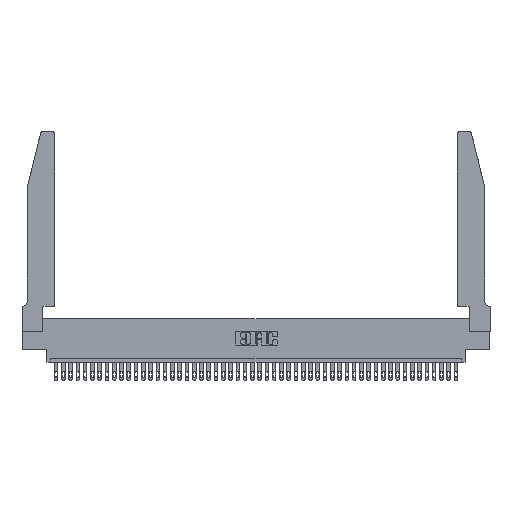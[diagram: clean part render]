
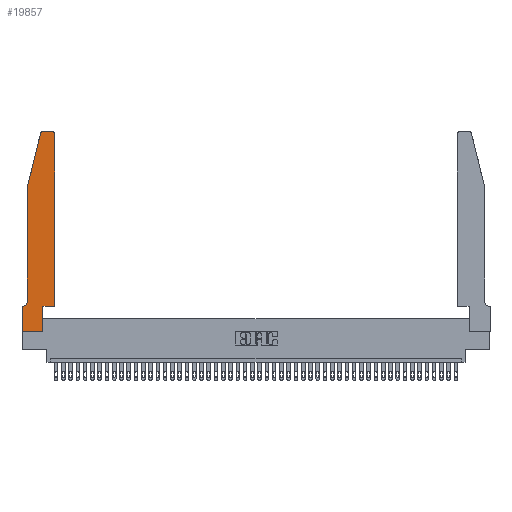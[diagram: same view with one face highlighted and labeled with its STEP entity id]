
A CAD part, top view. The second image highlights one B-rep face of the part: STEP entity #19857.
In plain terms, the highlighted planar face has unit normal (0, 0, 1).
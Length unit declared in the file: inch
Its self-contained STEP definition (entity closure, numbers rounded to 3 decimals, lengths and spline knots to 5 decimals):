
#42 = DIRECTION ( 'NONE',  ( -1., 0., 0. ) ) ;
#402 = CARTESIAN_POINT ( 'NONE',  ( 0.0755, 0.35, 0.37 ) ) ;
#424 = EDGE_CURVE ( 'NONE', #44941, #26855, #13581, .T. ) ;
#565 = EDGE_CURVE ( 'NONE', #4076, #39928, #29343, .T. ) ;
#1055 = CARTESIAN_POINT ( 'NONE',  ( 0., 0., 0.37 ) ) ;
#1721 = VERTEX_POINT ( 'NONE', #27410 ) ;
#1811 = CARTESIAN_POINT ( 'NONE',  ( 0.0055, 0.42, 0.37 ) ) ;
#3792 = ORIENTED_EDGE ( 'NONE', *, *, #565, .T. ) ;
#4076 = VERTEX_POINT ( 'NONE', #27846 ) ;
#5322 = DIRECTION ( 'NONE',  ( -1., 0., 0. ) ) ;
#5922 = VERTEX_POINT ( 'NONE', #16880 ) ;
#6200 = CARTESIAN_POINT ( 'NONE',  ( 0.0755, 2., 0.37 ) ) ;
#6797 = CARTESIAN_POINT ( 'NONE',  ( 0., 0., 0.37 ) ) ;
#7977 = DIRECTION ( 'NONE',  ( 0., 1., 0. ) ) ;
#7980 = LINE ( 'NONE', #35970, #43939 ) ;
#8084 = EDGE_LOOP ( 'NONE', ( #31897, #26178, #3792, #16799, #24186, #38973, #32315, #42271, #27465, #10610, #21210, #30016 ) ) ;
#8278 = DIRECTION ( 'NONE',  ( 0., 0., 1. ) ) ;
#8656 = CARTESIAN_POINT ( 'NONE',  ( 0.2865, 0., 0.37 ) ) ;
#9208 = FACE_OUTER_BOUND ( 'NONE', #8084, .T. ) ;
#9556 = VECTOR ( 'NONE', #25522, 39.37008 ) ;
#10610 = ORIENTED_EDGE ( 'NONE', *, *, #17469, .T. ) ;
#11180 = CARTESIAN_POINT ( 'NONE',  ( 0., 0.35, 0.37 ) ) ;
#11490 = CARTESIAN_POINT ( 'NONE',  ( 0., 0.35, 0.37 ) ) ;
#12446 = DIRECTION ( 'NONE',  ( -1., 0., 0. ) ) ;
#12644 = CIRCLE ( 'NONE', #36156, 0.03 ) ;
#13353 = DIRECTION ( 'NONE',  ( 0., -1., 0. ) ) ;
#13367 = VERTEX_POINT ( 'NONE', #11490 ) ;
#13550 = DIRECTION ( 'NONE',  ( 1., 0., 0. ) ) ;
#13581 = LINE ( 'NONE', #30031, #29385 ) ;
#14349 = DIRECTION ( 'NONE',  ( -0.239, -0.971, 0. ) ) ;
#15126 = DIRECTION ( 'NONE',  ( 0., 1., 0. ) ) ;
#15372 = CIRCLE ( 'NONE', #18150, 0.07 ) ;
#15380 = CARTESIAN_POINT ( 'NONE',  ( 0.0755, 2., 0.37 ) ) ;
#15788 = EDGE_CURVE ( 'NONE', #32384, #19058, #18793, .T. ) ;
#16799 = ORIENTED_EDGE ( 'NONE', *, *, #23053, .T. ) ;
#16880 = CARTESIAN_POINT ( 'NONE',  ( 0.2865, 0.35, 0.37 ) ) ;
#17407 = LINE ( 'NONE', #43301, #25046 ) ;
#17469 = EDGE_CURVE ( 'NONE', #5922, #43700, #27540, .T. ) ;
#18100 = EDGE_CURVE ( 'NONE', #21520, #44941, #12644, .T. ) ;
#18150 = AXIS2_PLACEMENT_3D ( 'NONE', #1811, #26254, #5322 ) ;
#18564 = CARTESIAN_POINT ( 'NONE',  ( 0.4505, 0.35, 0.37 ) ) ;
#18793 = LINE ( 'NONE', #1055, #9556 ) ;
#19058 = VERTEX_POINT ( 'NONE', #8656 ) ;
#19482 = LINE ( 'NONE', #6797, #43342 ) ;
#19632 = EDGE_CURVE ( 'NONE', #19058, #5922, #17407, .T. ) ;
#19857 = ADVANCED_FACE ( 'NONE', ( #9208 ), #25406, .T. ) ;
#20082 = AXIS2_PLACEMENT_3D ( 'NONE', #40966, #23455, #13550 ) ;
#21210 = ORIENTED_EDGE ( 'NONE', *, *, #23343, .T. ) ;
#21415 = CARTESIAN_POINT ( 'NONE',  ( 0.0055, 0.35, 0.37 ) ) ;
#21520 = VERTEX_POINT ( 'NONE', #23321 ) ;
#22359 = CARTESIAN_POINT ( 'NONE',  ( 0., 0., 0.37 ) ) ;
#22390 = DIRECTION ( 'NONE',  ( 0., -1., 0. ) ) ;
#23053 = EDGE_CURVE ( 'NONE', #39928, #1721, #25487, .T. ) ;
#23083 = VECTOR ( 'NONE', #29264, 39.37008 ) ;
#23321 = CARTESIAN_POINT ( 'NONE',  ( 0.4505, 2.72, 0.37 ) ) ;
#23343 = EDGE_CURVE ( 'NONE', #43700, #21520, #7980, .T. ) ;
#23455 = DIRECTION ( 'NONE',  ( 0., 0., 1. ) ) ;
#24186 = ORIENTED_EDGE ( 'NONE', *, *, #42506, .T. ) ;
#25046 = VECTOR ( 'NONE', #7977, 39.37008 ) ;
#25406 = PLANE ( 'NONE',  #39424 ) ;
#25487 = LINE ( 'NONE', #15380, #37453 ) ;
#25522 = DIRECTION ( 'NONE',  ( 1., 0., 0. ) ) ;
#26178 = ORIENTED_EDGE ( 'NONE', *, *, #28301, .T. ) ;
#26254 = DIRECTION ( 'NONE',  ( 0., 0., -1. ) ) ;
#26855 = VERTEX_POINT ( 'NONE', #32047 ) ;
#27380 = DIRECTION ( 'NONE',  ( 0., 0., 1. ) ) ;
#27410 = CARTESIAN_POINT ( 'NONE',  ( 0.0755, 0.42, 0.37 ) ) ;
#27465 = ORIENTED_EDGE ( 'NONE', *, *, #19632, .T. ) ;
#27540 = LINE ( 'NONE', #18564, #23083 ) ;
#27776 = CARTESIAN_POINT ( 'NONE',  ( 0.4505, 0.35, 0.37 ) ) ;
#27846 = CARTESIAN_POINT ( 'NONE',  ( 0.25487, 2.72718, 0.37 ) ) ;
#28301 = EDGE_CURVE ( 'NONE', #26855, #4076, #29218, .T. ) ;
#28796 = VECTOR ( 'NONE', #42, 39.37008 ) ;
#29218 = CIRCLE ( 'NONE', #20082, 0.03 ) ;
#29264 = DIRECTION ( 'NONE',  ( 1., 0., 0. ) ) ;
#29343 = LINE ( 'NONE', #31588, #42319 ) ;
#29385 = VECTOR ( 'NONE', #12446, 39.37008 ) ;
#30016 = ORIENTED_EDGE ( 'NONE', *, *, #18100, .T. ) ;
#30031 = CARTESIAN_POINT ( 'NONE',  ( 0.2605, 2.75, 0.37 ) ) ;
#30839 = DIRECTION ( 'NONE',  ( 1., 0., 0. ) ) ;
#31588 = CARTESIAN_POINT ( 'NONE',  ( 0.0755, 2., 0.37 ) ) ;
#31667 = EDGE_CURVE ( 'NONE', #34986, #13367, #37521, .T. ) ;
#31897 = ORIENTED_EDGE ( 'NONE', *, *, #424, .T. ) ;
#32047 = CARTESIAN_POINT ( 'NONE',  ( 0.284, 2.75, 0.37 ) ) ;
#32315 = ORIENTED_EDGE ( 'NONE', *, *, #39976, .T. ) ;
#32384 = VERTEX_POINT ( 'NONE', #22359 ) ;
#34986 = VERTEX_POINT ( 'NONE', #21415 ) ;
#35970 = CARTESIAN_POINT ( 'NONE',  ( 0.4505, 0.35, 0.37 ) ) ;
#36003 = DIRECTION ( 'NONE',  ( 1., 0., 0. ) ) ;
#36156 = AXIS2_PLACEMENT_3D ( 'NONE', #37676, #27380, #30839 ) ;
#37453 = VECTOR ( 'NONE', #22390, 39.37008 ) ;
#37521 = LINE ( 'NONE', #402, #28796 ) ;
#37676 = CARTESIAN_POINT ( 'NONE',  ( 0.4205, 2.72, 0.37 ) ) ;
#38973 = ORIENTED_EDGE ( 'NONE', *, *, #31667, .T. ) ;
#39424 = AXIS2_PLACEMENT_3D ( 'NONE', #11180, #8278, #36003 ) ;
#39928 = VERTEX_POINT ( 'NONE', #6200 ) ;
#39976 = EDGE_CURVE ( 'NONE', #13367, #32384, #19482, .T. ) ;
#40966 = CARTESIAN_POINT ( 'NONE',  ( 0.284, 2.72, 0.37 ) ) ;
#41496 = CARTESIAN_POINT ( 'NONE',  ( 0.4205, 2.75, 0.37 ) ) ;
#42271 = ORIENTED_EDGE ( 'NONE', *, *, #15788, .T. ) ;
#42319 = VECTOR ( 'NONE', #14349, 39.37008 ) ;
#42506 = EDGE_CURVE ( 'NONE', #1721, #34986, #15372, .T. ) ;
#43301 = CARTESIAN_POINT ( 'NONE',  ( 0.2865, 0.35, 0.37 ) ) ;
#43342 = VECTOR ( 'NONE', #13353, 39.37008 ) ;
#43700 = VERTEX_POINT ( 'NONE', #27776 ) ;
#43939 = VECTOR ( 'NONE', #15126, 39.37008 ) ;
#44941 = VERTEX_POINT ( 'NONE', #41496 ) ;
